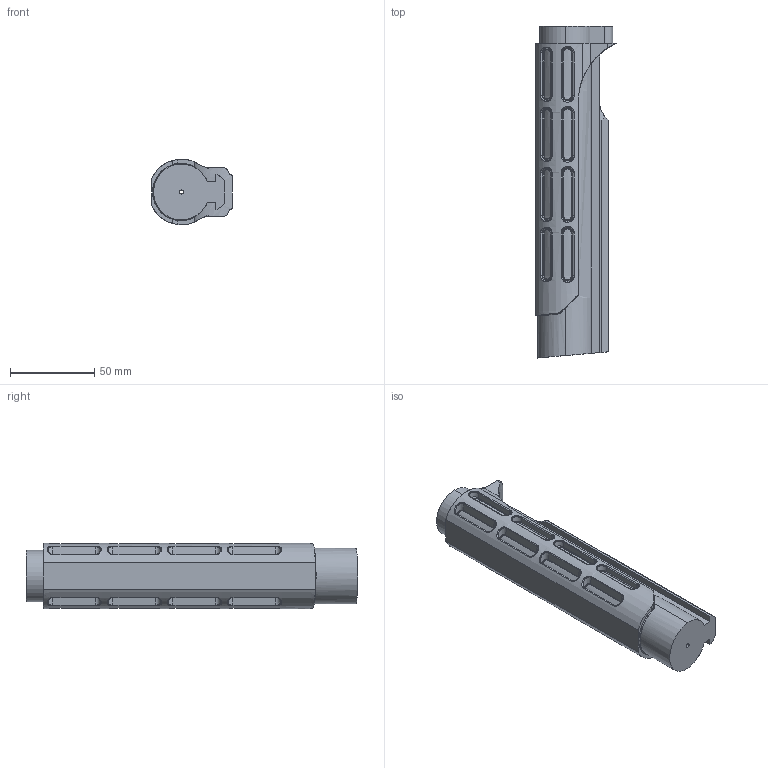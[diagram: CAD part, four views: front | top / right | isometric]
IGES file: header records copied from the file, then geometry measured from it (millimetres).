
Start section: SolidWorks IGES file using analytic representation for surfaces
Global section: file name: MKIIb Buffer tube.IGS; native system: SolidWorks 2012; preprocessor: SolidWorks 2012; author: Pld; date: 130926.052226; units: inch
Bounding box: 47.84 x 196.56 x 38.75 mm (x, y, z)
Surface area: 48967.7 mm2 (no closed solid volume)
Topology: 0 solids, 0 shells, 334 faces, 4074 edges, 4074 vertices
Faces by surface type: bspline 168, revolution 166
